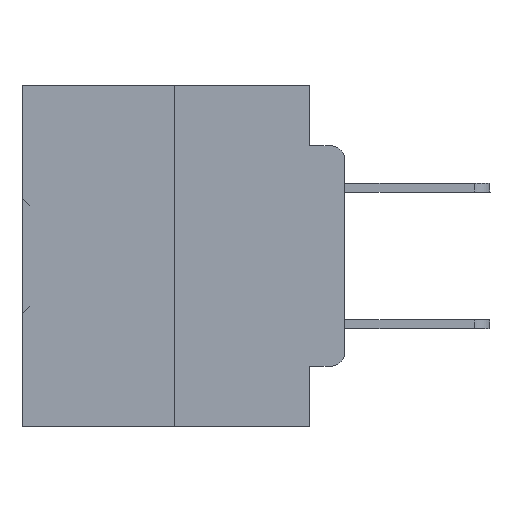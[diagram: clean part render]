
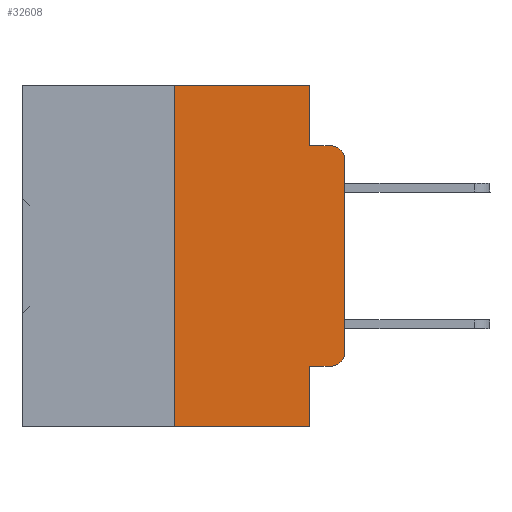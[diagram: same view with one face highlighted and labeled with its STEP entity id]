
A CAD part, left-side view. The second image highlights one B-rep face of the part: STEP entity #32608.
In plain terms, the highlighted planar face has unit normal (-1, 0, 0).
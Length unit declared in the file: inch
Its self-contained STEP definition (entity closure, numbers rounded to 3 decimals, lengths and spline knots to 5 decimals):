
#603 = LINE ( 'NONE', #14841, #15909 ) ;
#1622 = EDGE_CURVE ( 'NONE', #22351, #4082, #2873, .T. ) ;
#2178 = ORIENTED_EDGE ( 'NONE', *, *, #15511, .F. ) ;
#2248 = LINE ( 'NONE', #18946, #16578 ) ;
#2873 = LINE ( 'NONE', #18793, #24131 ) ;
#3112 = DIRECTION ( 'NONE',  ( -1., 0., 0. ) ) ;
#3721 = CARTESIAN_POINT ( 'NONE',  ( 0., 0.051, -0.0885 ) ) ;
#4082 = VERTEX_POINT ( 'NONE', #32386 ) ;
#5693 = DIRECTION ( 'NONE',  ( 0., -1., 0. ) ) ;
#5862 = AXIS2_PLACEMENT_3D ( 'NONE', #29725, #11806, #32702 ) ;
#5882 = VECTOR ( 'NONE', #14595, 39.37008 ) ;
#6864 = DIRECTION ( 'NONE',  ( 0., 0., -1. ) ) ;
#7475 = EDGE_CURVE ( 'NONE', #32757, #20730, #18353, .T. ) ;
#7968 = EDGE_CURVE ( 'NONE', #20886, #28005, #26756, .T. ) ;
#8161 = VECTOR ( 'NONE', #25624, 39.37008 ) ;
#8627 = PLANE ( 'NONE',  #5862 ) ;
#8988 = ORIENTED_EDGE ( 'NONE', *, *, #22818, .T. ) ;
#9369 = CARTESIAN_POINT ( 'NONE',  ( 0., 0.25, 0. ) ) ;
#9404 = ORIENTED_EDGE ( 'NONE', *, *, #30997, .F. ) ;
#9821 = FACE_OUTER_BOUND ( 'NONE', #11870, .T. ) ;
#9954 = CARTESIAN_POINT ( 'NONE',  ( 0., 0.02, -0.3915 ) ) ;
#9981 = DIRECTION ( 'NONE',  ( 0., -1., 0. ) ) ;
#11806 = DIRECTION ( 'NONE',  ( 1., 0., 0. ) ) ;
#11870 = EDGE_LOOP ( 'NONE', ( #25786, #12698, #2178, #12235, #35555, #9404, #27262, #27737, #8988, #20769 ) ) ;
#12235 = ORIENTED_EDGE ( 'NONE', *, *, #17777, .F. ) ;
#12374 = VERTEX_POINT ( 'NONE', #9369 ) ;
#12698 = ORIENTED_EDGE ( 'NONE', *, *, #7968, .T. ) ;
#13034 = DIRECTION ( 'NONE',  ( 0., 0., -1. ) ) ;
#14333 = CARTESIAN_POINT ( 'NONE',  ( 0., 0.25, -0.5 ) ) ;
#14442 = VERTEX_POINT ( 'NONE', #3721 ) ;
#14595 = DIRECTION ( 'NONE',  ( 0., 0., 1. ) ) ;
#14841 = CARTESIAN_POINT ( 'NONE',  ( 0., 0.051, -0.0885 ) ) ;
#15511 = EDGE_CURVE ( 'NONE', #14442, #28005, #603, .T. ) ;
#15769 = CARTESIAN_POINT ( 'NONE',  ( 0., 0.25, 0. ) ) ;
#15909 = VECTOR ( 'NONE', #20856, 39.37008 ) ;
#16578 = VECTOR ( 'NONE', #9981, 39.37008 ) ;
#17058 = EDGE_CURVE ( 'NONE', #12374, #21377, #26969, .T. ) ;
#17508 = CARTESIAN_POINT ( 'NONE',  ( 0., 0., 0. ) ) ;
#17777 = EDGE_CURVE ( 'NONE', #21377, #14442, #32060, .T. ) ;
#18126 = VECTOR ( 'NONE', #28406, 39.37008 ) ;
#18353 = CIRCLE ( 'NONE', #36445, 0.02 ) ;
#18793 = CARTESIAN_POINT ( 'NONE',  ( 0., 0.051, 0. ) ) ;
#18946 = CARTESIAN_POINT ( 'NONE',  ( 0., 0.473, -0.5 ) ) ;
#19743 = VECTOR ( 'NONE', #24755, 39.37008 ) ;
#20730 = VERTEX_POINT ( 'NONE', #25504 ) ;
#20769 = ORIENTED_EDGE ( 'NONE', *, *, #7475, .T. ) ;
#20856 = DIRECTION ( 'NONE',  ( 0., -1., 0. ) ) ;
#20886 = VERTEX_POINT ( 'NONE', #37995 ) ;
#21226 = CARTESIAN_POINT ( 'NONE',  ( 0., 0.02, -0.1085 ) ) ;
#21377 = VERTEX_POINT ( 'NONE', #25462 ) ;
#22351 = VERTEX_POINT ( 'NONE', #27443 ) ;
#22818 = EDGE_CURVE ( 'NONE', #22351, #32757, #23501, .T. ) ;
#22857 = LINE ( 'NONE', #17508, #5882 ) ;
#23501 = LINE ( 'NONE', #26755, #38285 ) ;
#24131 = VECTOR ( 'NONE', #6864, 39.37008 ) ;
#24232 = DIRECTION ( 'NONE',  ( 0., 0., -1. ) ) ;
#24755 = DIRECTION ( 'NONE',  ( 0., 0., 1. ) ) ;
#25462 = CARTESIAN_POINT ( 'NONE',  ( 0., 0.051, 0. ) ) ;
#25504 = CARTESIAN_POINT ( 'NONE',  ( 0., 0., -0.3915 ) ) ;
#25624 = DIRECTION ( 'NONE',  ( 0., 0., -1. ) ) ;
#25786 = ORIENTED_EDGE ( 'NONE', *, *, #34028, .T. ) ;
#26755 = CARTESIAN_POINT ( 'NONE',  ( 0., 0.051, -0.4115 ) ) ;
#26756 = CIRCLE ( 'NONE', #29074, 0.02 ) ;
#26969 = LINE ( 'NONE', #34325, #18126 ) ;
#27262 = ORIENTED_EDGE ( 'NONE', *, *, #30388, .T. ) ;
#27443 = CARTESIAN_POINT ( 'NONE',  ( 0., 0.051, -0.4115 ) ) ;
#27737 = ORIENTED_EDGE ( 'NONE', *, *, #1622, .F. ) ;
#28005 = VERTEX_POINT ( 'NONE', #28515 ) ;
#28406 = DIRECTION ( 'NONE',  ( 0., -1., 0. ) ) ;
#28515 = CARTESIAN_POINT ( 'NONE',  ( 0., 0.02, -0.0885 ) ) ;
#29074 = AXIS2_PLACEMENT_3D ( 'NONE', #21226, #3112, #24232 ) ;
#29565 = LINE ( 'NONE', #15769, #19743 ) ;
#29725 = CARTESIAN_POINT ( 'NONE',  ( 0., 0.473, 0. ) ) ;
#30253 = CARTESIAN_POINT ( 'NONE',  ( 0., 0.02, -0.4115 ) ) ;
#30388 = EDGE_CURVE ( 'NONE', #33971, #4082, #2248, .T. ) ;
#30933 = DIRECTION ( 'NONE',  ( -1., 0., 0. ) ) ;
#30997 = EDGE_CURVE ( 'NONE', #33971, #12374, #29565, .T. ) ;
#31464 = CARTESIAN_POINT ( 'NONE',  ( 0., 0.051, 0. ) ) ;
#32060 = LINE ( 'NONE', #31464, #8161 ) ;
#32386 = CARTESIAN_POINT ( 'NONE',  ( 0., 0.051, -0.5 ) ) ;
#32608 = ADVANCED_FACE ( 'NONE', ( #9821 ), #8627, .F. ) ;
#32702 = DIRECTION ( 'NONE',  ( 0., 0., -1. ) ) ;
#32757 = VERTEX_POINT ( 'NONE', #30253 ) ;
#33971 = VERTEX_POINT ( 'NONE', #14333 ) ;
#34028 = EDGE_CURVE ( 'NONE', #20730, #20886, #22857, .T. ) ;
#34325 = CARTESIAN_POINT ( 'NONE',  ( 0., 0.473, 0. ) ) ;
#35555 = ORIENTED_EDGE ( 'NONE', *, *, #17058, .F. ) ;
#36445 = AXIS2_PLACEMENT_3D ( 'NONE', #9954, #30933, #13034 ) ;
#37995 = CARTESIAN_POINT ( 'NONE',  ( 0., 0., -0.1085 ) ) ;
#38285 = VECTOR ( 'NONE', #5693, 39.37008 ) ;
